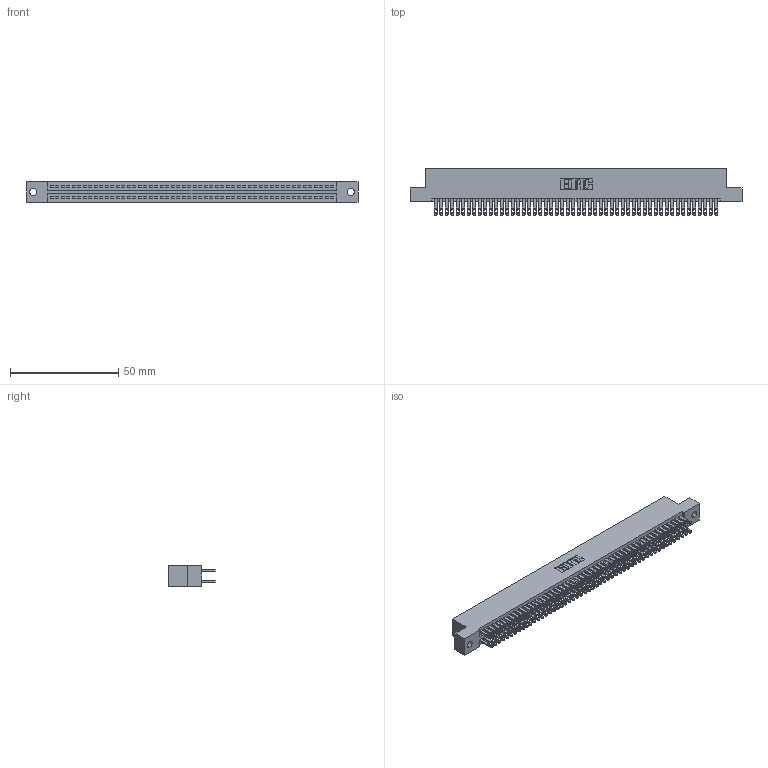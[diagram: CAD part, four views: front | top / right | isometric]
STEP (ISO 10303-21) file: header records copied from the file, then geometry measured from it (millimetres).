
FILE_DESCRIPTION (( 'STEP AP203' ), '1' );
FILE_NAME ('345-104-500-202.STEP', '2019-11-03T09:57:44', ( '' ), ( '' ), 'SwSTEP 2.0', 'SolidWorks 2016', '' );
FILE_SCHEMA (( 'CONFIG_CONTROL_DESIGN' ));
Length unit declared in the file: inch
Products named in the file (3): 345-292-001_345-293-100; 345 Part_Flush Mounting Lugs - 0.128 Dia; 345-104-500-202
Assembly tree (105 placements, depth 2):
  345-104-500-202
    345 Part_Flush Mounting Lugs - 0.128 Dia
    345-292-001_345-293-100  x104
Bounding box: 153.29 x 21.51 x 9.4 mm (x, y, z)
Volume: 15264.6 mm3; surface area: 23545.3 mm2
Topology: 105 solids, 105 shells, 4910 faces, 15005 edges, 10002 vertices
Faces by surface type: plane 2888, cylinder 2022
Entity records: 39387 total; most frequent: CARTESIAN_POINT 6592, ORIENTED_EDGE 6526, DIRECTION 5803, EDGE_CURVE 3263, VECTOR 2919, LINE 2919, VERTEX_POINT 2174, AXIS2_PLACEMENT_3D 1442
